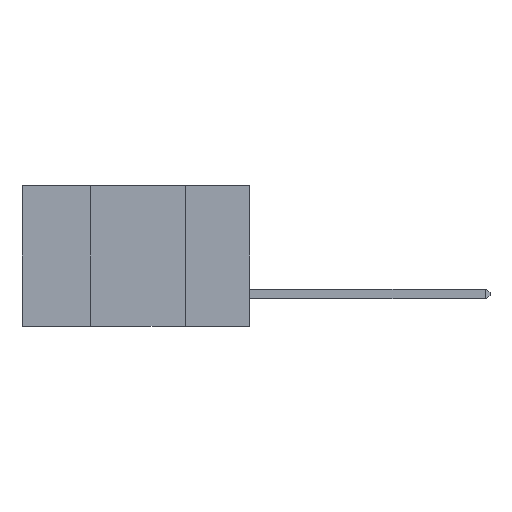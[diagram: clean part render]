
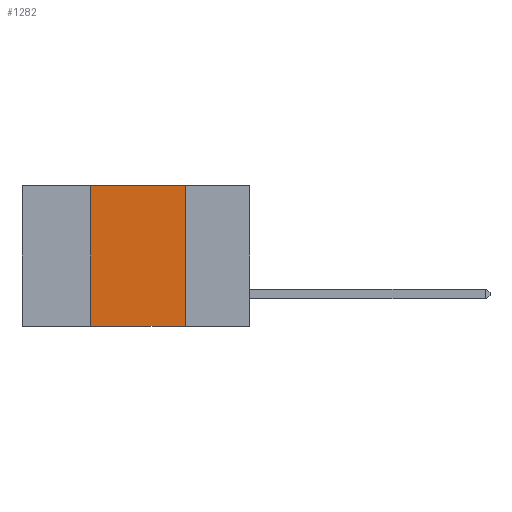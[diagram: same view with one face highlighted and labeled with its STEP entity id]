
A CAD part, left-side view. The second image highlights one B-rep face of the part: STEP entity #1282.
In plain terms, the highlighted planar face has unit normal (-1, 0, 0).
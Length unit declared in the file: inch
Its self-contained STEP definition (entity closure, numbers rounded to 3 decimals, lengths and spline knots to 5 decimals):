
#248 = ORIENTED_EDGE ( 'NONE', *, *, #4108, .T. ) ;
#457 = EDGE_CURVE ( 'NONE', #3086, #2390, #8491, .T. ) ;
#479 = ORIENTED_EDGE ( 'NONE', *, *, #1668, .F. ) ;
#1258 = ORIENTED_EDGE ( 'NONE', *, *, #457, .F. ) ;
#1282 = ADVANCED_FACE ( 'NONE', ( #6226 ), #7072, .F. ) ;
#1401 = ORIENTED_EDGE ( 'NONE', *, *, #5441, .F. ) ;
#1668 = EDGE_CURVE ( 'NONE', #6166, #3086, #2717, .T. ) ;
#1723 = CARTESIAN_POINT ( 'NONE',  ( 0., 0.17, 0. ) ) ;
#1771 = CARTESIAN_POINT ( 'NONE',  ( 0., 0.6, 0. ) ) ;
#2330 = AXIS2_PLACEMENT_3D ( 'NONE', #1771, #6915, #3614 ) ;
#2390 = VERTEX_POINT ( 'NONE', #1723 ) ;
#2717 = LINE ( 'NONE', #9467, #5314 ) ;
#3086 = VERTEX_POINT ( 'NONE', #5068 ) ;
#3138 = DIRECTION ( 'NONE',  ( 0., -1., 0. ) ) ;
#3179 = CARTESIAN_POINT ( 'NONE',  ( 0., 0.6, 0. ) ) ;
#3614 = DIRECTION ( 'NONE',  ( 0., 0., -1. ) ) ;
#3732 = EDGE_LOOP ( 'NONE', ( #1401, #1258, #479, #248 ) ) ;
#3806 = LINE ( 'NONE', #8111, #9452 ) ;
#4108 = EDGE_CURVE ( 'NONE', #6166, #9594, #3806, .T. ) ;
#4196 = CARTESIAN_POINT ( 'NONE',  ( 0., 0.42, -0.37 ) ) ;
#5068 = CARTESIAN_POINT ( 'NONE',  ( 0., 0.42, 0. ) ) ;
#5314 = VECTOR ( 'NONE', #9386, 39.37008 ) ;
#5441 = EDGE_CURVE ( 'NONE', #2390, #9594, #9422, .T. ) ;
#6166 = VERTEX_POINT ( 'NONE', #4196 ) ;
#6226 = FACE_OUTER_BOUND ( 'NONE', #3732, .T. ) ;
#6915 = DIRECTION ( 'NONE',  ( 1., 0., 0. ) ) ;
#7072 = PLANE ( 'NONE',  #2330 ) ;
#7174 = VECTOR ( 'NONE', #8761, 39.37008 ) ;
#7310 = DIRECTION ( 'NONE',  ( 0., -1., 0. ) ) ;
#8111 = CARTESIAN_POINT ( 'NONE',  ( 0., 0.6, -0.37 ) ) ;
#8491 = LINE ( 'NONE', #3179, #8705 ) ;
#8659 = CARTESIAN_POINT ( 'NONE',  ( 0., 0.17, -0.37 ) ) ;
#8705 = VECTOR ( 'NONE', #3138, 39.37008 ) ;
#8761 = DIRECTION ( 'NONE',  ( 0., 0., -1. ) ) ;
#9386 = DIRECTION ( 'NONE',  ( 0., 0., 1. ) ) ;
#9422 = LINE ( 'NONE', #10192, #7174 ) ;
#9452 = VECTOR ( 'NONE', #7310, 39.37008 ) ;
#9467 = CARTESIAN_POINT ( 'NONE',  ( 0., 0.42, 0. ) ) ;
#9594 = VERTEX_POINT ( 'NONE', #8659 ) ;
#10192 = CARTESIAN_POINT ( 'NONE',  ( 0., 0.17, 0. ) ) ;
